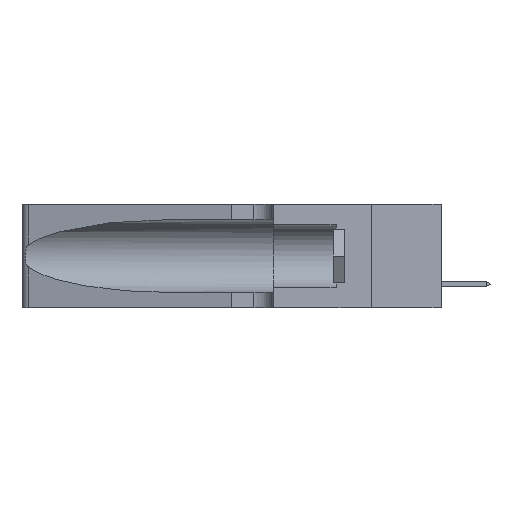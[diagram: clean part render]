
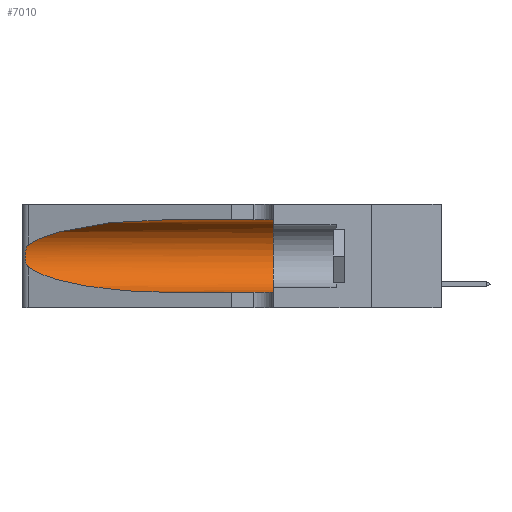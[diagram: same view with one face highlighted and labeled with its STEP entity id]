
A CAD part, left-side view. The second image highlights one B-rep face of the part: STEP entity #7010.
In plain terms, the highlighted cylindrical face has radius 3.308 mm (diameter 6.617 mm), a partial arc.
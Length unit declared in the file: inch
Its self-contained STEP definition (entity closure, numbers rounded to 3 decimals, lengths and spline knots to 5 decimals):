
#422 = CARTESIAN_POINT ( 'NONE',  ( 0.1305, 1.61858, 0.31525 ) ) ;
#821 = B_SPLINE_CURVE_WITH_KNOTS ( 'NONE', 3,
 ( #24286, #16546, #14521, #21391, #2117, #23977, #11958, #4574, #9396, #26441, #16866, #2317, #11851, #7150 ),
 .UNSPECIFIED., .F., .F.,
 ( 4, 2, 2, 2, 2, 2, 4 ),
 ( 0., 0.00027, 0.00053, 0.00107, 0.0016, 0.00187, 0.00214 ),
 .UNSPECIFIED. ) ;
#1467 = EDGE_CURVE ( 'NONE', #26100, #29220, #8978, .T. ) ;
#1801 = EDGE_CURVE ( 'NONE', #6293, #8489, #3340, .T. ) ;
#2027 = ORIENTED_EDGE ( 'NONE', *, *, #21709, .T. ) ;
#2117 = CARTESIAN_POINT ( 'NONE',  ( 0.25854, 1.2359, 0.20912 ) ) ;
#2317 = CARTESIAN_POINT ( 'NONE',  ( 0.25639, 1.23186, 0.15144 ) ) ;
#2657 = CARTESIAN_POINT ( 'NONE',  ( 0.18966, 0.96281, 0.31525 ) ) ;
#2749 = CARTESIAN_POINT ( 'NONE',  ( 0.25487, 1.22718, 0.22369 ) ) ;
#3340 =( BOUNDED_CURVE ( )  B_SPLINE_CURVE ( 3, ( #20903, #6360, #3938, #16161 ),
 .UNSPECIFIED., .F., .F. ) 
 B_SPLINE_CURVE_WITH_KNOTS ( ( 4, 4 ),
 ( 3.44316, 4.71239 ),
 .UNSPECIFIED. ) 
 CURVE ( )  GEOMETRIC_REPRESENTATION_ITEM ( )  RATIONAL_B_SPLINE_CURVE ( ( 1., 0.87, 0.87, 1. ) ) 
 REPRESENTATION_ITEM ( '' )  );
#3436 = ORIENTED_EDGE ( 'NONE', *, *, #1801, .T. ) ;
#3938 = CARTESIAN_POINT ( 'NONE',  ( 0.18966, 0.96281, 0.05475 ) ) ;
#4535 = LINE ( 'NONE', #26817, #26612 ) ;
#4574 = CARTESIAN_POINT ( 'NONE',  ( 0.26075, 1.23896, 0.178 ) ) ;
#5600 = AXIS2_PLACEMENT_3D ( 'NONE', #13705, #25819, #11349 ) ;
#6293 = VERTEX_POINT ( 'NONE', #25252 ) ;
#6360 = CARTESIAN_POINT ( 'NONE',  ( 0.2373, 1.15595, 0.08982 ) ) ;
#6560 = CARTESIAN_POINT ( 'NONE',  ( 0.1305, 0.72297, 0.05475 ) ) ;
#6876 = FACE_OUTER_BOUND ( 'NONE', #7372, .T. ) ;
#7010 = ADVANCED_FACE ( 'NONE', ( #6876 ), #12998, .F. ) ;
#7150 = CARTESIAN_POINT ( 'NONE',  ( 0.25487, 1.22718, 0.14631 ) ) ;
#7372 = EDGE_LOOP ( 'NONE', ( #15258, #14429, #3436, #2027, #16028, #17924 ) ) ;
#8434 = VERTEX_POINT ( 'NONE', #29147 ) ;
#8489 = VERTEX_POINT ( 'NONE', #6560 ) ;
#8978 =( BOUNDED_CURVE ( )  B_SPLINE_CURVE ( 3, ( #23919, #2657, #17273, #2749 ),
 .UNSPECIFIED., .F., .F. ) 
 B_SPLINE_CURVE_WITH_KNOTS ( ( 4, 4 ),
 ( 1.5708, 2.84003 ),
 .UNSPECIFIED. ) 
 CURVE ( )  GEOMETRIC_REPRESENTATION_ITEM ( )  RATIONAL_B_SPLINE_CURVE ( ( 1., 0.87, 0.87, 1. ) ) 
 REPRESENTATION_ITEM ( '' )  );
#9269 = EDGE_CURVE ( 'NONE', #9949, #8434, #17009, .T. ) ;
#9396 = CARTESIAN_POINT ( 'NONE',  ( 0.26017, 1.23833, 0.17102 ) ) ;
#9949 = VERTEX_POINT ( 'NONE', #28631 ) ;
#11349 = DIRECTION ( 'NONE',  ( 0., 0., 1. ) ) ;
#11851 = CARTESIAN_POINT ( 'NONE',  ( 0.25555, 1.22993, 0.14849 ) ) ;
#11958 = CARTESIAN_POINT ( 'NONE',  ( 0.26075, 1.23896, 0.19203 ) ) ;
#12922 = CARTESIAN_POINT ( 'NONE',  ( 0.1305, 1.61858, 0.185 ) ) ;
#12998 = CYLINDRICAL_SURFACE ( 'NONE', #22018, 0.13025 ) ;
#13660 = LINE ( 'NONE', #422, #27714 ) ;
#13705 = CARTESIAN_POINT ( 'NONE',  ( 0.1305, 0.35, 0.185 ) ) ;
#13805 = EDGE_CURVE ( 'NONE', #26100, #9949, #13660, .T. ) ;
#14429 = ORIENTED_EDGE ( 'NONE', *, *, #25461, .T. ) ;
#14521 = CARTESIAN_POINT ( 'NONE',  ( 0.25639, 1.23184, 0.21858 ) ) ;
#15258 = ORIENTED_EDGE ( 'NONE', *, *, #1467, .T. ) ;
#16028 = ORIENTED_EDGE ( 'NONE', *, *, #9269, .F. ) ;
#16161 = CARTESIAN_POINT ( 'NONE',  ( 0.1305, 0.72297, 0.05475 ) ) ;
#16546 = CARTESIAN_POINT ( 'NONE',  ( 0.25555, 1.22994, 0.2215 ) ) ;
#16866 = CARTESIAN_POINT ( 'NONE',  ( 0.25789, 1.23486, 0.15765 ) ) ;
#17009 = CIRCLE ( 'NONE', #5600, 0.13025 ) ;
#17273 = CARTESIAN_POINT ( 'NONE',  ( 0.2373, 1.15595, 0.28018 ) ) ;
#17924 = ORIENTED_EDGE ( 'NONE', *, *, #13805, .F. ) ;
#19857 = DIRECTION ( 'NONE',  ( 0., -1., 0. ) ) ;
#20113 = CARTESIAN_POINT ( 'NONE',  ( 0.1305, 0.72297, 0.31525 ) ) ;
#20903 = CARTESIAN_POINT ( 'NONE',  ( 0.25487, 1.22718, 0.14631 ) ) ;
#21221 = CARTESIAN_POINT ( 'NONE',  ( 0.25487, 1.22718, 0.22369 ) ) ;
#21391 = CARTESIAN_POINT ( 'NONE',  ( 0.25787, 1.23484, 0.2124 ) ) ;
#21709 = EDGE_CURVE ( 'NONE', #8489, #8434, #4535, .T. ) ;
#22018 = AXIS2_PLACEMENT_3D ( 'NONE', #12922, #25242, #29809 ) ;
#23919 = CARTESIAN_POINT ( 'NONE',  ( 0.1305, 0.72297, 0.31525 ) ) ;
#23977 = CARTESIAN_POINT ( 'NONE',  ( 0.26018, 1.23835, 0.19895 ) ) ;
#24286 = CARTESIAN_POINT ( 'NONE',  ( 0.25487, 1.22718, 0.22369 ) ) ;
#24949 = DIRECTION ( 'NONE',  ( 0., -1., 0. ) ) ;
#25242 = DIRECTION ( 'NONE',  ( 0., -1., 0. ) ) ;
#25252 = CARTESIAN_POINT ( 'NONE',  ( 0.25487, 1.22718, 0.14631 ) ) ;
#25461 = EDGE_CURVE ( 'NONE', #29220, #6293, #821, .T. ) ;
#25819 = DIRECTION ( 'NONE',  ( 0., 1., 0. ) ) ;
#26100 = VERTEX_POINT ( 'NONE', #20113 ) ;
#26441 = CARTESIAN_POINT ( 'NONE',  ( 0.25856, 1.23593, 0.16098 ) ) ;
#26612 = VECTOR ( 'NONE', #19857, 39.37008 ) ;
#26817 = CARTESIAN_POINT ( 'NONE',  ( 0.1305, 1.61858, 0.05475 ) ) ;
#27714 = VECTOR ( 'NONE', #24949, 39.37008 ) ;
#28631 = CARTESIAN_POINT ( 'NONE',  ( 0.1305, 0.35, 0.31525 ) ) ;
#29147 = CARTESIAN_POINT ( 'NONE',  ( 0.1305, 0.35, 0.05475 ) ) ;
#29220 = VERTEX_POINT ( 'NONE', #21221 ) ;
#29809 = DIRECTION ( 'NONE',  ( 0., 0., -1. ) ) ;
